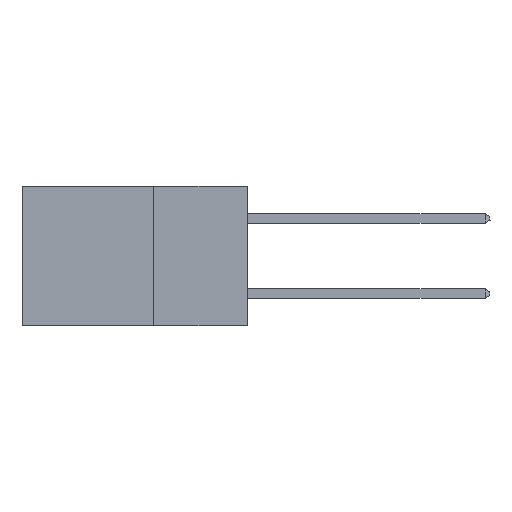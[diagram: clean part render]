
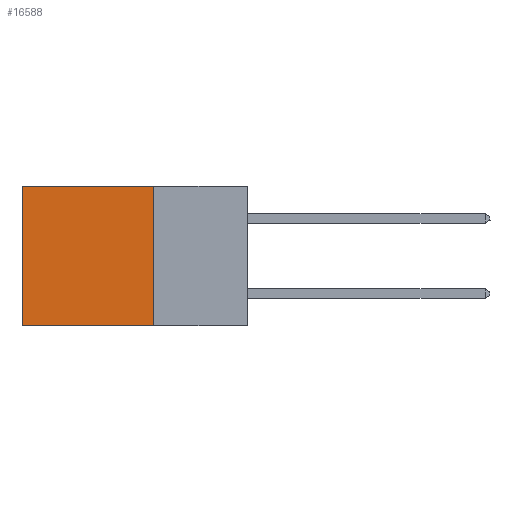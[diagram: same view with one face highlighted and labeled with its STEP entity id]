
A CAD part, left-side view. The second image highlights one B-rep face of the part: STEP entity #16588.
In plain terms, the highlighted planar face has unit normal (-1, 0, 0).
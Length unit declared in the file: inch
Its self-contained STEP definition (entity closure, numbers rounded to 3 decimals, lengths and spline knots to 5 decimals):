
#675 = DIRECTION ( 'NONE',  ( 0., 1., 0. ) ) ;
#956 = ORIENTED_EDGE ( 'NONE', *, *, #29073, .T. ) ;
#1535 = EDGE_CURVE ( 'NONE', #28138, #28723, #23394, .T. ) ;
#2709 = CARTESIAN_POINT ( 'NONE',  ( 0.298, 0.25, 0. ) ) ;
#2773 = DIRECTION ( 'NONE',  ( 0., 0., -1. ) ) ;
#3013 = VECTOR ( 'NONE', #31755, 39.37008 ) ;
#3779 = LINE ( 'NONE', #6836, #3013 ) ;
#4523 = CARTESIAN_POINT ( 'NONE',  ( 0.298, 0.6, 0. ) ) ;
#4692 = DIRECTION ( 'NONE',  ( 0., 1., 0. ) ) ;
#5195 = VECTOR ( 'NONE', #4692, 39.37008 ) ;
#5728 = DIRECTION ( 'NONE',  ( 0., 0., -1. ) ) ;
#6836 = CARTESIAN_POINT ( 'NONE',  ( 0.298, 0.25, 0. ) ) ;
#7724 = ORIENTED_EDGE ( 'NONE', *, *, #8348, .F. ) ;
#8023 = FACE_OUTER_BOUND ( 'NONE', #30610, .T. ) ;
#8348 = EDGE_CURVE ( 'NONE', #23695, #31392, #3779, .T. ) ;
#10129 = DIRECTION ( 'NONE',  ( 1., 0., 0. ) ) ;
#10226 = AXIS2_PLACEMENT_3D ( 'NONE', #22559, #10129, #2773 ) ;
#10878 = EDGE_CURVE ( 'NONE', #31392, #28723, #11789, .T. ) ;
#11345 = ORIENTED_EDGE ( 'NONE', *, *, #10878, .F. ) ;
#11789 = LINE ( 'NONE', #24666, #5195 ) ;
#15416 = PLANE ( 'NONE',  #10226 ) ;
#16267 = CARTESIAN_POINT ( 'NONE',  ( 0.298, 0.25, -0.37 ) ) ;
#16588 = ADVANCED_FACE ( 'NONE', ( #8023 ), #15416, .F. ) ;
#20165 = VECTOR ( 'NONE', #675, 39.37008 ) ;
#20532 = CARTESIAN_POINT ( 'NONE',  ( 0.298, 0.6, 0. ) ) ;
#22400 = ORIENTED_EDGE ( 'NONE', *, *, #1535, .T. ) ;
#22559 = CARTESIAN_POINT ( 'NONE',  ( 0.298, 0.25, 0. ) ) ;
#22759 = CARTESIAN_POINT ( 'NONE',  ( 0.298, 0.6, -0.37 ) ) ;
#23394 = LINE ( 'NONE', #20532, #23750 ) ;
#23695 = VERTEX_POINT ( 'NONE', #2709 ) ;
#23750 = VECTOR ( 'NONE', #5728, 39.37008 ) ;
#24666 = CARTESIAN_POINT ( 'NONE',  ( 0.298, 0.25, -0.37 ) ) ;
#28138 = VERTEX_POINT ( 'NONE', #4523 ) ;
#28723 = VERTEX_POINT ( 'NONE', #22759 ) ;
#29073 = EDGE_CURVE ( 'NONE', #23695, #28138, #29374, .T. ) ;
#29374 = LINE ( 'NONE', #30431, #20165 ) ;
#30431 = CARTESIAN_POINT ( 'NONE',  ( 0.298, 0.25, 0. ) ) ;
#30610 = EDGE_LOOP ( 'NONE', ( #22400, #11345, #7724, #956 ) ) ;
#31392 = VERTEX_POINT ( 'NONE', #16267 ) ;
#31755 = DIRECTION ( 'NONE',  ( 0., 0., -1. ) ) ;
